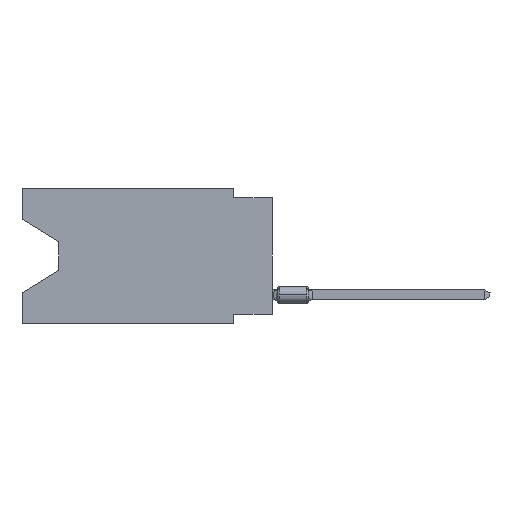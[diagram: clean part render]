
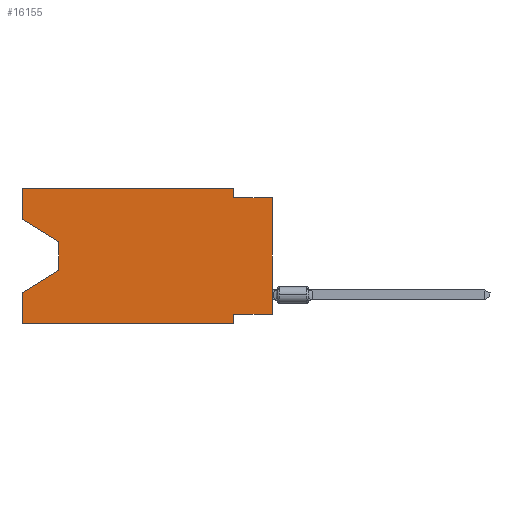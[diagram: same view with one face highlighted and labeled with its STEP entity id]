
A CAD part, left-side view. The second image highlights one B-rep face of the part: STEP entity #16155.
In plain terms, the highlighted planar face has unit normal (-1, 0, 0).
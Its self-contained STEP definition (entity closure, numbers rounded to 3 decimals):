
#832 = VERTEX_POINT ( 'NONE', #5956 ) ;
#1508 = LINE ( 'NONE', #10199, #113018 ) ;
#1735 = VECTOR ( 'NONE', #49037, 1000. ) ;
#2718 = VECTOR ( 'NONE', #14837, 1000. ) ;
#5510 = CARTESIAN_POINT ( 'NONE',  ( 0., 0., 0. ) ) ;
#5956 = CARTESIAN_POINT ( 'NONE',  ( 0., 2.54, 0. ) ) ;
#7584 = CARTESIAN_POINT ( 'NONE',  ( 0., 16.383, 0. ) ) ;
#7876 = EDGE_CURVE ( 'NONE', #92275, #20419, #41213, .T. ) ;
#7992 = ORIENTED_EDGE ( 'NONE', *, *, #70735, .F. ) ;
#8132 = ORIENTED_EDGE ( 'NONE', *, *, #57172, .T. ) ;
#8260 = DIRECTION ( 'NONE',  ( 0., 0., -1. ) ) ;
#9571 = DIRECTION ( 'NONE',  ( 0., -1., 0. ) ) ;
#9871 = EDGE_CURVE ( 'NONE', #93577, #97692, #19533, .T. ) ;
#10199 = CARTESIAN_POINT ( 'NONE',  ( 0., 16.383, -8.89 ) ) ;
#10310 = CARTESIAN_POINT ( 'NONE',  ( 0., 16.383, -8.89 ) ) ;
#10853 = CARTESIAN_POINT ( 'NONE',  ( 0., 16.383, -2.038 ) ) ;
#13280 = VECTOR ( 'NONE', #9571, 1000. ) ;
#13857 = ORIENTED_EDGE ( 'NONE', *, *, #15466, .F. ) ;
#14837 = DIRECTION ( 'NONE',  ( 0., 0., -1. ) ) ;
#15466 = EDGE_CURVE ( 'NONE', #49974, #55263, #56510, .T. ) ;
#15553 = ORIENTED_EDGE ( 'NONE', *, *, #9871, .F. ) ;
#16155 = ADVANCED_FACE ( 'NONE', ( #113799 ), #69638, .F. ) ;
#16753 = DIRECTION ( 'NONE',  ( 0., 0.855, -0.519 ) ) ;
#19533 = LINE ( 'NONE', #90357, #103532 ) ;
#19535 = VECTOR ( 'NONE', #8260, 1000. ) ;
#20419 = VERTEX_POINT ( 'NONE', #23319 ) ;
#21018 = CARTESIAN_POINT ( 'NONE',  ( 0., 16.383, 0. ) ) ;
#21139 = EDGE_LOOP ( 'NONE', ( #66520, #108834, #41199, #15553, #109665, #83629, #113220, #8132, #13857, #56049, #7992, #77979 ) ) ;
#22161 = DIRECTION ( 'NONE',  ( 0., -1., 0. ) ) ;
#23319 = CARTESIAN_POINT ( 'NONE',  ( 0., 2.54, -8.89 ) ) ;
#23609 = EDGE_CURVE ( 'NONE', #93577, #20419, #1508, .T. ) ;
#24467 = CARTESIAN_POINT ( 'NONE',  ( 0., 16.383, 0. ) ) ;
#26481 = DIRECTION ( 'NONE',  ( 0., -1., 0. ) ) ;
#27223 = VECTOR ( 'NONE', #49900, 1000. ) ;
#29690 = CARTESIAN_POINT ( 'NONE',  ( 0., 0., -0.635 ) ) ;
#30292 = LINE ( 'NONE', #21018, #75210 ) ;
#33404 = LINE ( 'NONE', #49653, #2718 ) ;
#34444 = CARTESIAN_POINT ( 'NONE',  ( 0., 2.54, -0.635 ) ) ;
#35570 = CARTESIAN_POINT ( 'NONE',  ( 0., 13.97, -3.505 ) ) ;
#37470 = EDGE_CURVE ( 'NONE', #113477, #91120, #113919, .T. ) ;
#38370 = CARTESIAN_POINT ( 'NONE',  ( 0., 13.97, -3.505 ) ) ;
#41199 = ORIENTED_EDGE ( 'NONE', *, *, #65722, .T. ) ;
#41213 = LINE ( 'NONE', #66751, #27223 ) ;
#44271 = CARTESIAN_POINT ( 'NONE',  ( 0., 2.54, -8.255 ) ) ;
#46249 = DIRECTION ( 'NONE',  ( 0., 0., 1. ) ) ;
#49037 = DIRECTION ( 'NONE',  ( 0., 0., 1. ) ) ;
#49653 = CARTESIAN_POINT ( 'NONE',  ( 0., 2.54, 0. ) ) ;
#49900 = DIRECTION ( 'NONE',  ( 0., 0., -1. ) ) ;
#49974 = VERTEX_POINT ( 'NONE', #34444 ) ;
#49982 = CARTESIAN_POINT ( 'NONE',  ( 0., 0., -8.255 ) ) ;
#49984 = CARTESIAN_POINT ( 'NONE',  ( 0., 0., -8.255 ) ) ;
#50524 = DIRECTION ( 'NONE',  ( 0., 0., -1. ) ) ;
#52850 = CARTESIAN_POINT ( 'NONE',  ( 0., 13.97, -5.385 ) ) ;
#55155 = VECTOR ( 'NONE', #63649, 1000. ) ;
#55263 = VERTEX_POINT ( 'NONE', #29690 ) ;
#56049 = ORIENTED_EDGE ( 'NONE', *, *, #81149, .F. ) ;
#56510 = LINE ( 'NONE', #98936, #13280 ) ;
#57172 = EDGE_CURVE ( 'NONE', #65065, #55263, #93177, .T. ) ;
#58174 = VECTOR ( 'NONE', #22161, 1000. ) ;
#58539 = CARTESIAN_POINT ( 'NONE',  ( 0., 16.383, -2.038 ) ) ;
#60861 = VECTOR ( 'NONE', #111540, 1000. ) ;
#61531 = VERTEX_POINT ( 'NONE', #58539 ) ;
#63649 = DIRECTION ( 'NONE',  ( 0., -0.855, -0.519 ) ) ;
#64965 = EDGE_CURVE ( 'NONE', #61531, #78339, #30292, .T. ) ;
#65065 = VERTEX_POINT ( 'NONE', #49984 ) ;
#65722 = EDGE_CURVE ( 'NONE', #91120, #97692, #96856, .T. ) ;
#66520 = ORIENTED_EDGE ( 'NONE', *, *, #84715, .T. ) ;
#66751 = CARTESIAN_POINT ( 'NONE',  ( 0., 2.54, -8.89 ) ) ;
#69638 = PLANE ( 'NONE',  #77961 ) ;
#70735 = EDGE_CURVE ( 'NONE', #78339, #832, #76652, .T. ) ;
#72368 = LINE ( 'NONE', #10853, #55155 ) ;
#73191 = CARTESIAN_POINT ( 'NONE',  ( 0., 16.383, -6.852 ) ) ;
#75210 = VECTOR ( 'NONE', #108691, 1000. ) ;
#76652 = LINE ( 'NONE', #112082, #58174 ) ;
#77790 = DIRECTION ( 'NONE',  ( 1., 0., 0. ) ) ;
#77961 = AXIS2_PLACEMENT_3D ( 'NONE', #7584, #77790, #50524 ) ;
#77979 = ORIENTED_EDGE ( 'NONE', *, *, #64965, .F. ) ;
#78339 = VERTEX_POINT ( 'NONE', #24467 ) ;
#81149 = EDGE_CURVE ( 'NONE', #832, #49974, #33404, .T. ) ;
#83629 = ORIENTED_EDGE ( 'NONE', *, *, #7876, .F. ) ;
#84715 = EDGE_CURVE ( 'NONE', #61531, #113477, #72368, .T. ) ;
#86832 = EDGE_CURVE ( 'NONE', #65065, #92275, #101113, .T. ) ;
#90357 = CARTESIAN_POINT ( 'NONE',  ( 0., 16.383, 0. ) ) ;
#91120 = VERTEX_POINT ( 'NONE', #52850 ) ;
#92275 = VERTEX_POINT ( 'NONE', #44271 ) ;
#93177 = LINE ( 'NONE', #5510, #1735 ) ;
#93577 = VERTEX_POINT ( 'NONE', #10310 ) ;
#96856 = LINE ( 'NONE', #114272, #106556 ) ;
#97692 = VERTEX_POINT ( 'NONE', #73191 ) ;
#98936 = CARTESIAN_POINT ( 'NONE',  ( 0., 0., -0.635 ) ) ;
#101113 = LINE ( 'NONE', #49982, #60861 ) ;
#103532 = VECTOR ( 'NONE', #46249, 1000. ) ;
#106556 = VECTOR ( 'NONE', #16753, 1000. ) ;
#108691 = DIRECTION ( 'NONE',  ( 0., 0., 1. ) ) ;
#108834 = ORIENTED_EDGE ( 'NONE', *, *, #37470, .T. ) ;
#109665 = ORIENTED_EDGE ( 'NONE', *, *, #23609, .T. ) ;
#111540 = DIRECTION ( 'NONE',  ( 0., 1., 0. ) ) ;
#112082 = CARTESIAN_POINT ( 'NONE',  ( 0., 16.383, 0. ) ) ;
#113018 = VECTOR ( 'NONE', #26481, 1000. ) ;
#113220 = ORIENTED_EDGE ( 'NONE', *, *, #86832, .F. ) ;
#113477 = VERTEX_POINT ( 'NONE', #38370 ) ;
#113799 = FACE_OUTER_BOUND ( 'NONE', #21139, .T. ) ;
#113919 = LINE ( 'NONE', #35570, #19535 ) ;
#114272 = CARTESIAN_POINT ( 'NONE',  ( 0., 13.97, -5.385 ) ) ;
